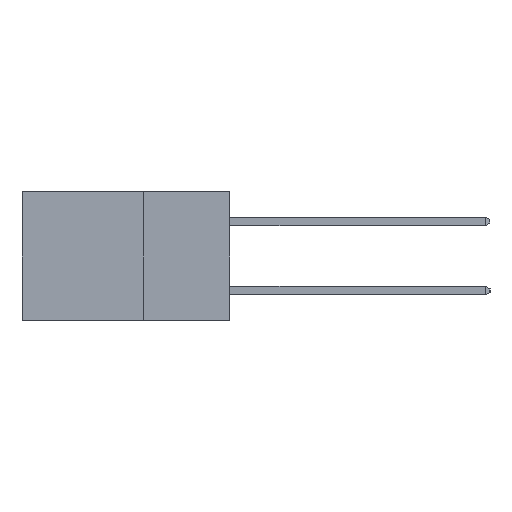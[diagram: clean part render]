
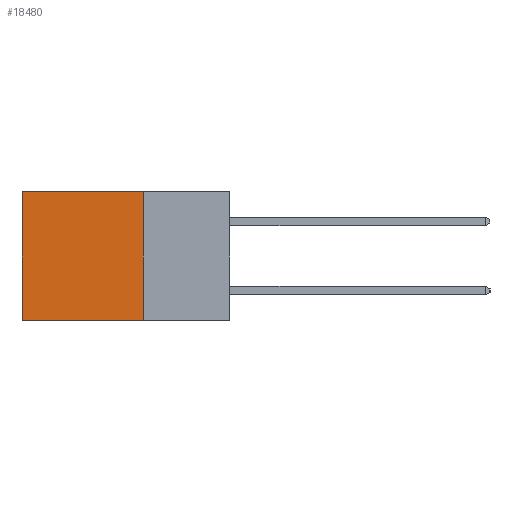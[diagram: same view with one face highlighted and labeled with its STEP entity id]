
A CAD part, left-side view. The second image highlights one B-rep face of the part: STEP entity #18480.
In plain terms, the highlighted planar face has unit normal (-1, 0, 0).
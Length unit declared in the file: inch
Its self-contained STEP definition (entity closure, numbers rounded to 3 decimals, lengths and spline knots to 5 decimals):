
#43 = EDGE_CURVE ( 'NONE', #3691, #475, #9211, .T. ) ;
#475 = VERTEX_POINT ( 'NONE', #6592 ) ;
#1061 = CARTESIAN_POINT ( 'NONE',  ( 0.2615, 0.6, -0.37 ) ) ;
#1185 = VECTOR ( 'NONE', #18719, 39.37008 ) ;
#2697 = CARTESIAN_POINT ( 'NONE',  ( 0.2615, 0.25, 0. ) ) ;
#2766 = EDGE_CURVE ( 'NONE', #5247, #12316, #17516, .T. ) ;
#2798 = EDGE_LOOP ( 'NONE', ( #9788, #5447, #8244, #12889 ) ) ;
#3038 = CARTESIAN_POINT ( 'NONE',  ( 0.2615, 0.25, -0.37 ) ) ;
#3369 = CARTESIAN_POINT ( 'NONE',  ( 0.2615, 0.6, -0.37 ) ) ;
#3691 = VERTEX_POINT ( 'NONE', #2697 ) ;
#4684 = FACE_OUTER_BOUND ( 'NONE', #2798, .T. ) ;
#5247 = VERTEX_POINT ( 'NONE', #9148 ) ;
#5447 = ORIENTED_EDGE ( 'NONE', *, *, #2766, .F. ) ;
#5457 = PLANE ( 'NONE',  #16114 ) ;
#6249 = VECTOR ( 'NONE', #8146, 39.37008 ) ;
#6592 = CARTESIAN_POINT ( 'NONE',  ( 0.2615, 0.6, 0. ) ) ;
#7099 = VECTOR ( 'NONE', #13006, 39.37008 ) ;
#8146 = DIRECTION ( 'NONE',  ( 0., 1., 0. ) ) ;
#8244 = ORIENTED_EDGE ( 'NONE', *, *, #10753, .F. ) ;
#8440 = DIRECTION ( 'NONE',  ( 1., 0., 0. ) ) ;
#8858 = CARTESIAN_POINT ( 'NONE',  ( 0.2615, 0.25, -0.37 ) ) ;
#9148 = CARTESIAN_POINT ( 'NONE',  ( 0.2615, 0.25, -0.37 ) ) ;
#9211 = LINE ( 'NONE', #14006, #1185 ) ;
#9788 = ORIENTED_EDGE ( 'NONE', *, *, #16231, .T. ) ;
#10753 = EDGE_CURVE ( 'NONE', #3691, #5247, #12551, .T. ) ;
#11625 = VECTOR ( 'NONE', #16135, 39.37008 ) ;
#12316 = VERTEX_POINT ( 'NONE', #3369 ) ;
#12551 = LINE ( 'NONE', #8858, #11625 ) ;
#12889 = ORIENTED_EDGE ( 'NONE', *, *, #43, .T. ) ;
#13006 = DIRECTION ( 'NONE',  ( 0., 0., -1. ) ) ;
#14006 = CARTESIAN_POINT ( 'NONE',  ( 0.2615, 0.25, 0. ) ) ;
#16114 = AXIS2_PLACEMENT_3D ( 'NONE', #17208, #8440, #18680 ) ;
#16135 = DIRECTION ( 'NONE',  ( 0., 0., -1. ) ) ;
#16231 = EDGE_CURVE ( 'NONE', #475, #12316, #18328, .T. ) ;
#17208 = CARTESIAN_POINT ( 'NONE',  ( 0.2615, 0.25, -0.37 ) ) ;
#17516 = LINE ( 'NONE', #3038, #6249 ) ;
#18328 = LINE ( 'NONE', #1061, #7099 ) ;
#18480 = ADVANCED_FACE ( 'NONE', ( #4684 ), #5457, .F. ) ;
#18680 = DIRECTION ( 'NONE',  ( 0., 0., -1. ) ) ;
#18719 = DIRECTION ( 'NONE',  ( 0., 1., 0. ) ) ;
